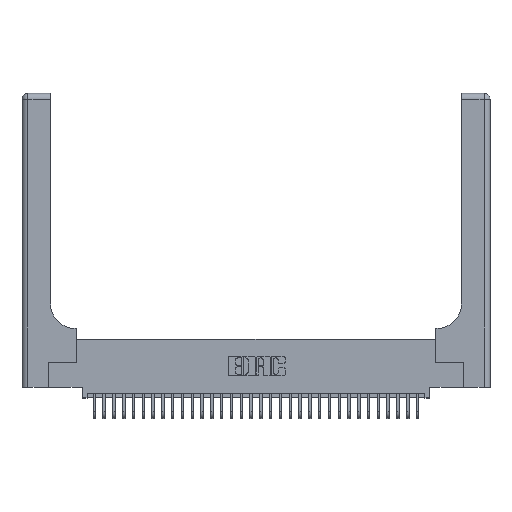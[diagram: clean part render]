
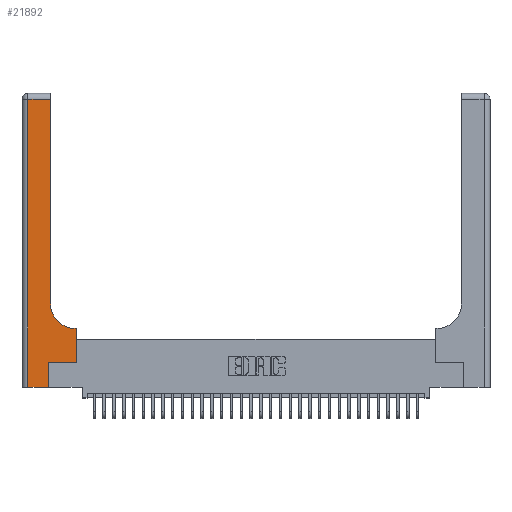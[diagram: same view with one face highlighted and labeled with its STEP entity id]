
A CAD part, top view. The second image highlights one B-rep face of the part: STEP entity #21892.
In plain terms, the highlighted planar face has unit normal (0, 0, 1).
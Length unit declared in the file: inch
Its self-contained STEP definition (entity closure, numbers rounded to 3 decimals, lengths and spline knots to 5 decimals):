
#267 = ORIENTED_EDGE ( 'NONE', *, *, #29605, .T. ) ;
#579 = ORIENTED_EDGE ( 'NONE', *, *, #5805, .T. ) ;
#1164 = EDGE_LOOP ( 'NONE', ( #579, #11300, #7908, #2710, #6157, #20331, #267, #29827, #7387 ) ) ;
#1585 = LINE ( 'NONE', #21754, #29316 ) ;
#1653 = VECTOR ( 'NONE', #31360, 39.37008 ) ;
#1969 = CARTESIAN_POINT ( 'NONE',  ( 0.2915, 2.94, 0.37 ) ) ;
#2558 = VECTOR ( 'NONE', #24829, 39.37008 ) ;
#2710 = ORIENTED_EDGE ( 'NONE', *, *, #17777, .T. ) ;
#3834 = VERTEX_POINT ( 'NONE', #8067 ) ;
#3872 = CARTESIAN_POINT ( 'NONE',  ( 0.269, 0.25, 0.37 ) ) ;
#4544 = CARTESIAN_POINT ( 'NONE',  ( 0.5585, 0.25, 0.37 ) ) ;
#5481 = CARTESIAN_POINT ( 'NONE',  ( 0., 3., 0.37 ) ) ;
#5765 = VECTOR ( 'NONE', #13828, 39.37008 ) ;
#5805 = EDGE_CURVE ( 'NONE', #24584, #14567, #24643, .T. ) ;
#6157 = ORIENTED_EDGE ( 'NONE', *, *, #7556, .T. ) ;
#6469 = VECTOR ( 'NONE', #12515, 39.37008 ) ;
#6574 = VERTEX_POINT ( 'NONE', #22559 ) ;
#6720 = AXIS2_PLACEMENT_3D ( 'NONE', #5481, #26821, #7815 ) ;
#7387 = ORIENTED_EDGE ( 'NONE', *, *, #32174, .T. ) ;
#7556 = EDGE_CURVE ( 'NONE', #29327, #24511, #27023, .T. ) ;
#7815 = DIRECTION ( 'NONE',  ( -1., 0., 0. ) ) ;
#7908 = ORIENTED_EDGE ( 'NONE', *, *, #15184, .T. ) ;
#7943 = CARTESIAN_POINT ( 'NONE',  ( 0.5415, 0.85, 0.37 ) ) ;
#8067 = CARTESIAN_POINT ( 'NONE',  ( 0.06, 2.94, 0.37 ) ) ;
#8315 = CARTESIAN_POINT ( 'NONE',  ( 0.2915, 3., 0.37 ) ) ;
#9755 = CARTESIAN_POINT ( 'NONE',  ( 0., 0., 0.37 ) ) ;
#11093 = EDGE_CURVE ( 'NONE', #6574, #24093, #34230, .T. ) ;
#11300 = ORIENTED_EDGE ( 'NONE', *, *, #15032, .T. ) ;
#12111 = LINE ( 'NONE', #4544, #19235 ) ;
#12515 = DIRECTION ( 'NONE',  ( 0., 1., 0. ) ) ;
#13329 = PLANE ( 'NONE',  #6720 ) ;
#13828 = DIRECTION ( 'NONE',  ( 0., 1., 0. ) ) ;
#13950 = VERTEX_POINT ( 'NONE', #27963 ) ;
#14364 = CARTESIAN_POINT ( 'NONE',  ( 0.5415, 0.6, 0.37 ) ) ;
#14567 = VERTEX_POINT ( 'NONE', #1969 ) ;
#15032 = EDGE_CURVE ( 'NONE', #14567, #3834, #21445, .T. ) ;
#15184 = EDGE_CURVE ( 'NONE', #3834, #31010, #31114, .T. ) ;
#15249 = DIRECTION ( 'NONE',  ( -1., 0., 0. ) ) ;
#15630 = CARTESIAN_POINT ( 'NONE',  ( 0.06, 0., 0.37 ) ) ;
#16273 = DIRECTION ( 'NONE',  ( 0., 0., -1. ) ) ;
#17777 = EDGE_CURVE ( 'NONE', #31010, #29327, #22695, .T. ) ;
#17778 = DIRECTION ( 'NONE',  ( 0., 1., 0. ) ) ;
#19083 = EDGE_CURVE ( 'NONE', #24511, #13950, #1585, .T. ) ;
#19235 = VECTOR ( 'NONE', #17778, 39.37008 ) ;
#19533 = CARTESIAN_POINT ( 'NONE',  ( 0.06, 3., 0.37 ) ) ;
#20331 = ORIENTED_EDGE ( 'NONE', *, *, #19083, .T. ) ;
#20353 = VECTOR ( 'NONE', #15249, 39.37008 ) ;
#21445 = LINE ( 'NONE', #27292, #2558 ) ;
#21754 = CARTESIAN_POINT ( 'NONE',  ( 0.269, 0.25, 0.37 ) ) ;
#21892 = ADVANCED_FACE ( 'NONE', ( #22383 ), #13329, .F. ) ;
#22276 = CARTESIAN_POINT ( 'NONE',  ( 0.269, 0., 0.37 ) ) ;
#22383 = FACE_OUTER_BOUND ( 'NONE', #1164, .T. ) ;
#22559 = CARTESIAN_POINT ( 'NONE',  ( 0.5585, 0.6, 0.37 ) ) ;
#22695 = LINE ( 'NONE', #9755, #1653 ) ;
#23974 = VECTOR ( 'NONE', #33592, 39.37008 ) ;
#24093 = VERTEX_POINT ( 'NONE', #14364 ) ;
#24511 = VERTEX_POINT ( 'NONE', #3872 ) ;
#24584 = VERTEX_POINT ( 'NONE', #33162 ) ;
#24643 = LINE ( 'NONE', #8315, #5765 ) ;
#24829 = DIRECTION ( 'NONE',  ( -1., 0., 0. ) ) ;
#26453 = CIRCLE ( 'NONE', #26909, 0.25 ) ;
#26821 = DIRECTION ( 'NONE',  ( 0., 0., -1. ) ) ;
#26909 = AXIS2_PLACEMENT_3D ( 'NONE', #7943, #16273, #29677 ) ;
#27023 = LINE ( 'NONE', #31764, #6469 ) ;
#27263 = DIRECTION ( 'NONE',  ( 1., 0., 0. ) ) ;
#27292 = CARTESIAN_POINT ( 'NONE',  ( 0., 2.94, 0.37 ) ) ;
#27963 = CARTESIAN_POINT ( 'NONE',  ( 0.5585, 0.25, 0.37 ) ) ;
#28644 = CARTESIAN_POINT ( 'NONE',  ( 0.2915, 0.6, 0.37 ) ) ;
#29316 = VECTOR ( 'NONE', #27263, 39.37008 ) ;
#29327 = VERTEX_POINT ( 'NONE', #22276 ) ;
#29605 = EDGE_CURVE ( 'NONE', #13950, #6574, #12111, .T. ) ;
#29677 = DIRECTION ( 'NONE',  ( 1., 0., 0. ) ) ;
#29827 = ORIENTED_EDGE ( 'NONE', *, *, #11093, .T. ) ;
#31010 = VERTEX_POINT ( 'NONE', #15630 ) ;
#31114 = LINE ( 'NONE', #19533, #23974 ) ;
#31360 = DIRECTION ( 'NONE',  ( 1., 0., 0. ) ) ;
#31764 = CARTESIAN_POINT ( 'NONE',  ( 0.269, 0., 0.37 ) ) ;
#32174 = EDGE_CURVE ( 'NONE', #24093, #24584, #26453, .T. ) ;
#33162 = CARTESIAN_POINT ( 'NONE',  ( 0.2915, 0.85, 0.37 ) ) ;
#33592 = DIRECTION ( 'NONE',  ( 0., -1., 0. ) ) ;
#34230 = LINE ( 'NONE', #28644, #20353 ) ;
